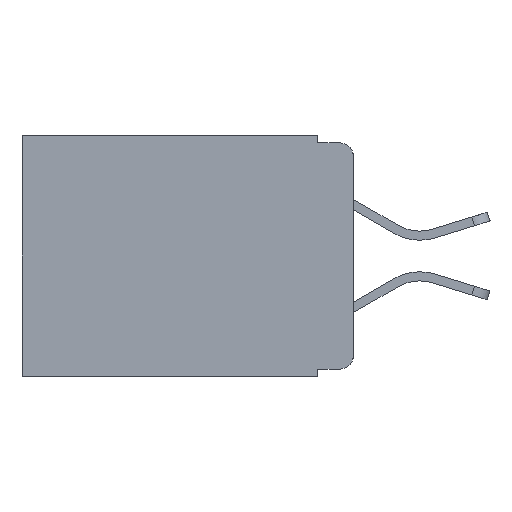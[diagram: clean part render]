
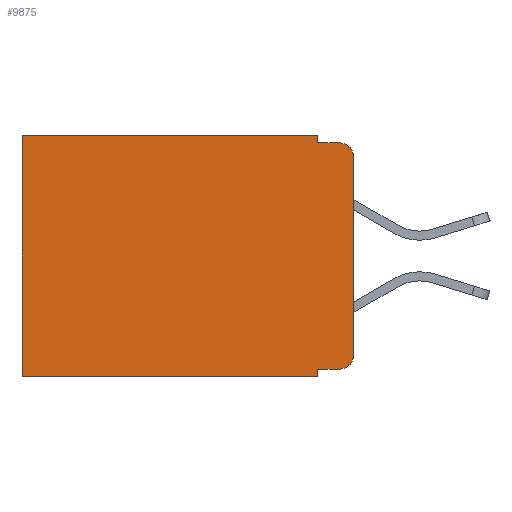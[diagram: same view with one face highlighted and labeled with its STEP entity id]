
A CAD part, left-side view. The second image highlights one B-rep face of the part: STEP entity #9875.
In plain terms, the highlighted planar face has unit normal (-1, 0, 0).
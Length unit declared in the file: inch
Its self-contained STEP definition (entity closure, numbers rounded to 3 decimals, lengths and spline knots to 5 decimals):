
#60 = VECTOR ( 'NONE', #2883, 39.37008 ) ;
#205 = AXIS2_PLACEMENT_3D ( 'NONE', #10586, #4572, #11545 ) ;
#417 = LINE ( 'NONE', #5383, #1213 ) ;
#432 = LINE ( 'NONE', #8099, #11609 ) ;
#575 = FACE_OUTER_BOUND ( 'NONE', #5545, .T. ) ;
#1086 = EDGE_CURVE ( 'NONE', #7253, #3216, #2102, .T. ) ;
#1171 = EDGE_CURVE ( 'NONE', #2926, #7253, #10944, .T. ) ;
#1213 = VECTOR ( 'NONE', #1321, 39.37008 ) ;
#1288 = DIRECTION ( 'NONE',  ( 0., 0., -1. ) ) ;
#1321 = DIRECTION ( 'NONE',  ( 0., -1., 0. ) ) ;
#1619 = VERTEX_POINT ( 'NONE', #8113 ) ;
#1915 = AXIS2_PLACEMENT_3D ( 'NONE', #9789, #5050, #7047 ) ;
#1941 = ORIENTED_EDGE ( 'NONE', *, *, #3882, .T. ) ;
#2090 = EDGE_CURVE ( 'NONE', #12604, #1619, #417, .T. ) ;
#2102 = LINE ( 'NONE', #4935, #60 ) ;
#2140 = LINE ( 'NONE', #9008, #8378 ) ;
#2386 = LINE ( 'NONE', #5354, #12077 ) ;
#2632 = VERTEX_POINT ( 'NONE', #3312 ) ;
#2883 = DIRECTION ( 'NONE',  ( 0., 1., 0. ) ) ;
#2926 = VERTEX_POINT ( 'NONE', #2945 ) ;
#2945 = CARTESIAN_POINT ( 'NONE',  ( 0.298, 0.051, -0.333 ) ) ;
#3171 = DIRECTION ( 'NONE',  ( 0., 0., -1. ) ) ;
#3216 = VERTEX_POINT ( 'NONE', #4777 ) ;
#3237 = VERTEX_POINT ( 'NONE', #11496 ) ;
#3312 = CARTESIAN_POINT ( 'NONE',  ( 0.298, 0.02, -0.333 ) ) ;
#3527 = EDGE_CURVE ( 'NONE', #3237, #3216, #2386, .T. ) ;
#3614 = ORIENTED_EDGE ( 'NONE', *, *, #6767, .T. ) ;
#3650 = CARTESIAN_POINT ( 'NONE',  ( 0.298, 0.051, -0.343 ) ) ;
#3761 = ORIENTED_EDGE ( 'NONE', *, *, #8449, .F. ) ;
#3849 = CIRCLE ( 'NONE', #10188, 0.02 ) ;
#3882 = EDGE_CURVE ( 'NONE', #2926, #2632, #432, .T. ) ;
#3996 = CARTESIAN_POINT ( 'NONE',  ( 0.298, 0.051, 0. ) ) ;
#4572 = DIRECTION ( 'NONE',  ( 1., 0., 0. ) ) ;
#4677 = EDGE_CURVE ( 'NONE', #2632, #5339, #5826, .T. ) ;
#4777 = CARTESIAN_POINT ( 'NONE',  ( 0.298, 0.473, -0.343 ) ) ;
#4850 = ORIENTED_EDGE ( 'NONE', *, *, #2090, .F. ) ;
#4935 = CARTESIAN_POINT ( 'NONE',  ( 0.298, 0., -0.343 ) ) ;
#5050 = DIRECTION ( 'NONE',  ( -1., 0., 0. ) ) ;
#5221 = DIRECTION ( 'NONE',  ( 0., -1., 0. ) ) ;
#5312 = ORIENTED_EDGE ( 'NONE', *, *, #1086, .F. ) ;
#5339 = VERTEX_POINT ( 'NONE', #7644 ) ;
#5354 = CARTESIAN_POINT ( 'NONE',  ( 0.298, 0.473, 0. ) ) ;
#5383 = CARTESIAN_POINT ( 'NONE',  ( 0.298, 0.051, -0.01 ) ) ;
#5545 = EDGE_LOOP ( 'NONE', ( #3761, #3614, #4850, #12549, #11403, #10857, #5312, #5954, #1941, #8289 ) ) ;
#5681 = CARTESIAN_POINT ( 'NONE',  ( 0.298, 0.051, 0. ) ) ;
#5826 = CIRCLE ( 'NONE', #1915, 0.02 ) ;
#5954 = ORIENTED_EDGE ( 'NONE', *, *, #1171, .F. ) ;
#6027 = DIRECTION ( 'NONE',  ( 0., 0., -1. ) ) ;
#6152 = EDGE_CURVE ( 'NONE', #10171, #3237, #11239, .T. ) ;
#6326 = DIRECTION ( 'NONE',  ( -1., 0., 0. ) ) ;
#6767 = EDGE_CURVE ( 'NONE', #10275, #1619, #3849, .T. ) ;
#6781 = LINE ( 'NONE', #5681, #12223 ) ;
#6873 = EDGE_CURVE ( 'NONE', #10171, #12604, #6781, .T. ) ;
#7047 = DIRECTION ( 'NONE',  ( 0., 0., -1. ) ) ;
#7253 = VERTEX_POINT ( 'NONE', #3650 ) ;
#7349 = DIRECTION ( 'NONE',  ( 0., 0., -1. ) ) ;
#7363 = VECTOR ( 'NONE', #7491, 39.37008 ) ;
#7477 = DIRECTION ( 'NONE',  ( 0., 0., -1. ) ) ;
#7491 = DIRECTION ( 'NONE',  ( 0., 1., 0. ) ) ;
#7644 = CARTESIAN_POINT ( 'NONE',  ( 0.298, 0., -0.313 ) ) ;
#8099 = CARTESIAN_POINT ( 'NONE',  ( 0.298, 0.051, -0.333 ) ) ;
#8113 = CARTESIAN_POINT ( 'NONE',  ( 0.298, 0.02, -0.01 ) ) ;
#8289 = ORIENTED_EDGE ( 'NONE', *, *, #4677, .T. ) ;
#8378 = VECTOR ( 'NONE', #3171, 39.37008 ) ;
#8416 = PLANE ( 'NONE',  #205 ) ;
#8449 = EDGE_CURVE ( 'NONE', #10275, #5339, #2140, .T. ) ;
#9008 = CARTESIAN_POINT ( 'NONE',  ( 0.298, 0., 0. ) ) ;
#9170 = CARTESIAN_POINT ( 'NONE',  ( 0.298, 0., -0.03 ) ) ;
#9405 = CARTESIAN_POINT ( 'NONE',  ( 0.298, 0., 0. ) ) ;
#9789 = CARTESIAN_POINT ( 'NONE',  ( 0.298, 0.02, -0.313 ) ) ;
#9875 = ADVANCED_FACE ( 'NONE', ( #575 ), #8416, .F. ) ;
#10171 = VERTEX_POINT ( 'NONE', #3996 ) ;
#10188 = AXIS2_PLACEMENT_3D ( 'NONE', #11166, #6326, #7349 ) ;
#10275 = VERTEX_POINT ( 'NONE', #9170 ) ;
#10469 = CARTESIAN_POINT ( 'NONE',  ( 0.298, 0.051, -0.01 ) ) ;
#10586 = CARTESIAN_POINT ( 'NONE',  ( 0.298, 0., 0. ) ) ;
#10857 = ORIENTED_EDGE ( 'NONE', *, *, #3527, .T. ) ;
#10944 = LINE ( 'NONE', #11957, #11944 ) ;
#11166 = CARTESIAN_POINT ( 'NONE',  ( 0.298, 0.02, -0.03 ) ) ;
#11239 = LINE ( 'NONE', #9405, #7363 ) ;
#11403 = ORIENTED_EDGE ( 'NONE', *, *, #6152, .T. ) ;
#11496 = CARTESIAN_POINT ( 'NONE',  ( 0.298, 0.473, 0. ) ) ;
#11545 = DIRECTION ( 'NONE',  ( 0., 0., -1. ) ) ;
#11609 = VECTOR ( 'NONE', #5221, 39.37008 ) ;
#11944 = VECTOR ( 'NONE', #6027, 39.37008 ) ;
#11957 = CARTESIAN_POINT ( 'NONE',  ( 0.298, 0.051, 0. ) ) ;
#12077 = VECTOR ( 'NONE', #1288, 39.37008 ) ;
#12223 = VECTOR ( 'NONE', #7477, 39.37008 ) ;
#12549 = ORIENTED_EDGE ( 'NONE', *, *, #6873, .F. ) ;
#12604 = VERTEX_POINT ( 'NONE', #10469 ) ;
